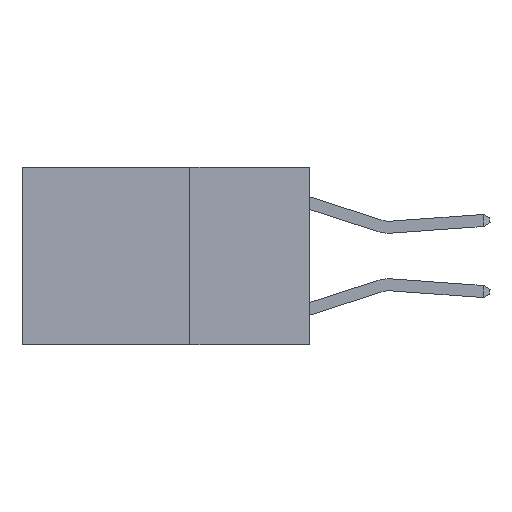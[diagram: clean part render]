
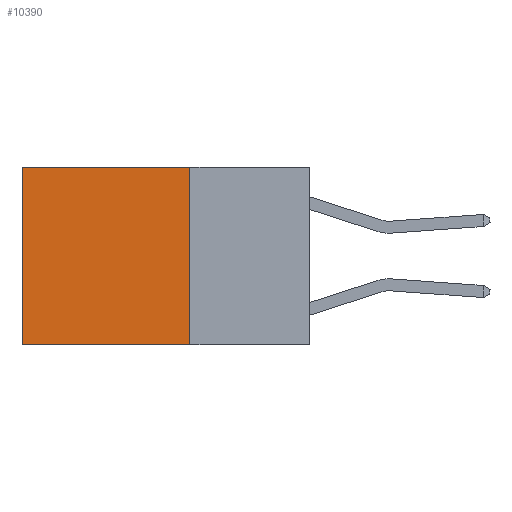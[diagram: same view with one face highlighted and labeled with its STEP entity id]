
A CAD part, left-side view. The second image highlights one B-rep face of the part: STEP entity #10390.
In plain terms, the highlighted planar face has unit normal (-1, 0, 0).
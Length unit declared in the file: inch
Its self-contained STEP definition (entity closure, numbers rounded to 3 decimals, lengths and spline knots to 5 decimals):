
#423 = AXIS2_PLACEMENT_3D ( 'NONE', #1144, #6660, #3799 ) ;
#525 = VERTEX_POINT ( 'NONE', #2162 ) ;
#756 = CARTESIAN_POINT ( 'NONE',  ( 0.2625, 0.25, 0. ) ) ;
#1144 = CARTESIAN_POINT ( 'NONE',  ( 0.2625, 0.25, 0. ) ) ;
#1812 = VECTOR ( 'NONE', #11875, 39.37008 ) ;
#1822 = ORIENTED_EDGE ( 'NONE', *, *, #3493, .F. ) ;
#1943 = CARTESIAN_POINT ( 'NONE',  ( 0.2625, 0.6, 0. ) ) ;
#2162 = CARTESIAN_POINT ( 'NONE',  ( 0.2625, 0.6, -0.37 ) ) ;
#2234 = VECTOR ( 'NONE', #7819, 39.37008 ) ;
#2589 = VECTOR ( 'NONE', #3432, 39.37008 ) ;
#3091 = VERTEX_POINT ( 'NONE', #3840 ) ;
#3432 = DIRECTION ( 'NONE',  ( 0., 0., -1. ) ) ;
#3493 = EDGE_CURVE ( 'NONE', #5557, #525, #4383, .T. ) ;
#3575 = ORIENTED_EDGE ( 'NONE', *, *, #10125, .T. ) ;
#3799 = DIRECTION ( 'NONE',  ( 0., 0., -1. ) ) ;
#3840 = CARTESIAN_POINT ( 'NONE',  ( 0.2625, 0.25, 0. ) ) ;
#4117 = CARTESIAN_POINT ( 'NONE',  ( 0.2625, 0.6, 0. ) ) ;
#4383 = LINE ( 'NONE', #8831, #7294 ) ;
#5557 = VERTEX_POINT ( 'NONE', #8736 ) ;
#6019 = DIRECTION ( 'NONE',  ( 0., 1., 0. ) ) ;
#6220 = EDGE_CURVE ( 'NONE', #10854, #525, #6921, .T. ) ;
#6547 = PLANE ( 'NONE',  #423 ) ;
#6660 = DIRECTION ( 'NONE',  ( 1., 0., 0. ) ) ;
#6921 = LINE ( 'NONE', #4117, #2234 ) ;
#7260 = ORIENTED_EDGE ( 'NONE', *, *, #10238, .F. ) ;
#7294 = VECTOR ( 'NONE', #6019, 39.37008 ) ;
#7819 = DIRECTION ( 'NONE',  ( 0., 0., -1. ) ) ;
#8586 = FACE_OUTER_BOUND ( 'NONE', #10169, .T. ) ;
#8736 = CARTESIAN_POINT ( 'NONE',  ( 0.2625, 0.25, -0.37 ) ) ;
#8795 = ORIENTED_EDGE ( 'NONE', *, *, #6220, .T. ) ;
#8831 = CARTESIAN_POINT ( 'NONE',  ( 0.2625, 0.25, -0.37 ) ) ;
#10125 = EDGE_CURVE ( 'NONE', #3091, #10854, #10997, .T. ) ;
#10169 = EDGE_LOOP ( 'NONE', ( #8795, #1822, #7260, #3575 ) ) ;
#10238 = EDGE_CURVE ( 'NONE', #3091, #5557, #11955, .T. ) ;
#10390 = ADVANCED_FACE ( 'NONE', ( #8586 ), #6547, .F. ) ;
#10854 = VERTEX_POINT ( 'NONE', #1943 ) ;
#10997 = LINE ( 'NONE', #756, #1812 ) ;
#11836 = CARTESIAN_POINT ( 'NONE',  ( 0.2625, 0.25, 0. ) ) ;
#11875 = DIRECTION ( 'NONE',  ( 0., 1., 0. ) ) ;
#11955 = LINE ( 'NONE', #11836, #2589 ) ;
